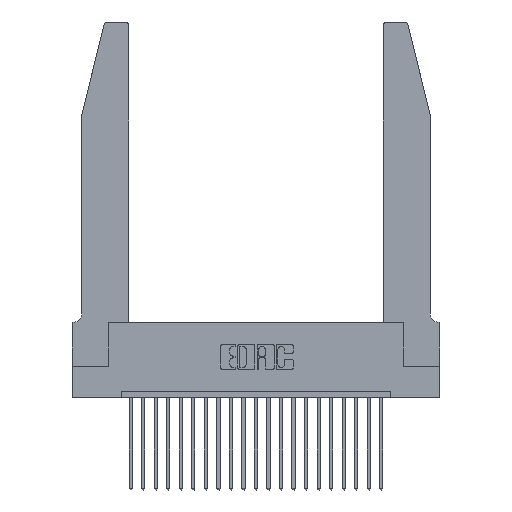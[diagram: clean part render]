
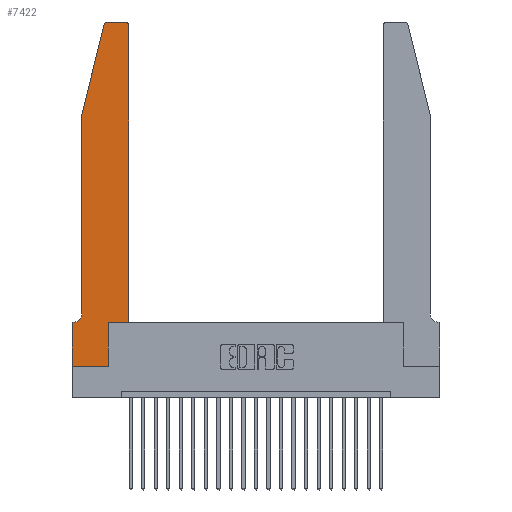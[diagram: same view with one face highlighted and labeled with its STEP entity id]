
A CAD part, top view. The second image highlights one B-rep face of the part: STEP entity #7422.
In plain terms, the highlighted planar face has unit normal (0, 0, 1).
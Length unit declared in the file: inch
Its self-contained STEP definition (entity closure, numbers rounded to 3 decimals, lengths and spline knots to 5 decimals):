
#168 = DIRECTION ( 'NONE',  ( 0., -1., 0. ) ) ;
#185 = VECTOR ( 'NONE', #168, 39.37008 ) ;
#1058 = CARTESIAN_POINT ( 'NONE',  ( 0., 0., 0.37 ) ) ;
#1091 = DIRECTION ( 'NONE',  ( 1., 0., 0. ) ) ;
#1201 = ORIENTED_EDGE ( 'NONE', *, *, #13110, .T. ) ;
#1692 = EDGE_CURVE ( 'NONE', #3059, #1806, #6596, .T. ) ;
#1806 = VERTEX_POINT ( 'NONE', #16091 ) ;
#1858 = CARTESIAN_POINT ( 'NONE',  ( 0.0055, 0.35, 0.37 ) ) ;
#1915 = VECTOR ( 'NONE', #3840, 39.37008 ) ;
#1952 = EDGE_LOOP ( 'NONE', ( #14640, #12118, #13056, #22120, #21061, #23394, #17642, #8916, #16453, #1201, #12430, #7201 ) ) ;
#1994 = AXIS2_PLACEMENT_3D ( 'NONE', #22771, #15600, #23003 ) ;
#2488 = EDGE_CURVE ( 'NONE', #17588, #18552, #19065, .T. ) ;
#2520 = AXIS2_PLACEMENT_3D ( 'NONE', #21531, #5009, #7047 ) ;
#3059 = VERTEX_POINT ( 'NONE', #19355 ) ;
#3170 = CIRCLE ( 'NONE', #3537, 0.03 ) ;
#3206 = VECTOR ( 'NONE', #23325, 39.37008 ) ;
#3537 = AXIS2_PLACEMENT_3D ( 'NONE', #4564, #6344, #1091 ) ;
#3687 = CARTESIAN_POINT ( 'NONE',  ( 0.2865, 0.35, 0.37 ) ) ;
#3840 = DIRECTION ( 'NONE',  ( -0.239, -0.971, 0. ) ) ;
#4564 = CARTESIAN_POINT ( 'NONE',  ( 0.284, 2.72, 0.37 ) ) ;
#4999 = LINE ( 'NONE', #12201, #185 ) ;
#5009 = DIRECTION ( 'NONE',  ( 0., 0., -1. ) ) ;
#5666 = DIRECTION ( 'NONE',  ( 1., 0., 0. ) ) ;
#5783 = PLANE ( 'NONE',  #11746 ) ;
#6344 = DIRECTION ( 'NONE',  ( 0., 0., 1. ) ) ;
#6596 = CIRCLE ( 'NONE', #1994, 0.03 ) ;
#6610 = VERTEX_POINT ( 'NONE', #14616 ) ;
#7047 = DIRECTION ( 'NONE',  ( -1., 0., 0. ) ) ;
#7201 = ORIENTED_EDGE ( 'NONE', *, *, #1692, .T. ) ;
#7284 = VERTEX_POINT ( 'NONE', #1858 ) ;
#7287 = CARTESIAN_POINT ( 'NONE',  ( 0.0755, 2., 0.37 ) ) ;
#7422 = ADVANCED_FACE ( 'NONE', ( #21648 ), #5783, .T. ) ;
#7629 = CARTESIAN_POINT ( 'NONE',  ( 0.2605, 2.75, 0.37 ) ) ;
#7743 = VECTOR ( 'NONE', #13198, 39.37008 ) ;
#8656 = LINE ( 'NONE', #7287, #1915 ) ;
#8835 = LINE ( 'NONE', #21524, #3206 ) ;
#8916 = ORIENTED_EDGE ( 'NONE', *, *, #15512, .T. ) ;
#9559 = CARTESIAN_POINT ( 'NONE',  ( 0., 0.35, 0.37 ) ) ;
#9866 = VECTOR ( 'NONE', #16115, 39.37008 ) ;
#10441 = CARTESIAN_POINT ( 'NONE',  ( 0.4505, 0.35, 0.37 ) ) ;
#10525 = EDGE_CURVE ( 'NONE', #16802, #6610, #4999, .T. ) ;
#11103 = EDGE_CURVE ( 'NONE', #19682, #16802, #8656, .T. ) ;
#11746 = AXIS2_PLACEMENT_3D ( 'NONE', #18501, #22245, #17152 ) ;
#12118 = ORIENTED_EDGE ( 'NONE', *, *, #17867, .T. ) ;
#12201 = CARTESIAN_POINT ( 'NONE',  ( 0.0755, 2., 0.37 ) ) ;
#12286 = CARTESIAN_POINT ( 'NONE',  ( 0.284, 2.75, 0.37 ) ) ;
#12384 = CARTESIAN_POINT ( 'NONE',  ( 0.0755, 0.35, 0.37 ) ) ;
#12430 = ORIENTED_EDGE ( 'NONE', *, *, #12512, .T. ) ;
#12512 = EDGE_CURVE ( 'NONE', #16644, #3059, #12854, .T. ) ;
#12854 = LINE ( 'NONE', #17814, #14546 ) ;
#12873 = CARTESIAN_POINT ( 'NONE',  ( 0.0755, 2., 0.37 ) ) ;
#12982 = CARTESIAN_POINT ( 'NONE',  ( 0.2865, 0., 0.37 ) ) ;
#13056 = ORIENTED_EDGE ( 'NONE', *, *, #11103, .T. ) ;
#13110 = EDGE_CURVE ( 'NONE', #13647, #16644, #8835, .T. ) ;
#13198 = DIRECTION ( 'NONE',  ( -1., 0., 0. ) ) ;
#13647 = VERTEX_POINT ( 'NONE', #14885 ) ;
#13722 = VECTOR ( 'NONE', #5666, 39.37008 ) ;
#13962 = LINE ( 'NONE', #7629, #7743 ) ;
#14505 = EDGE_CURVE ( 'NONE', #16985, #13647, #22277, .T. ) ;
#14546 = VECTOR ( 'NONE', #18055, 39.37008 ) ;
#14616 = CARTESIAN_POINT ( 'NONE',  ( 0.0755, 0.42, 0.37 ) ) ;
#14640 = ORIENTED_EDGE ( 'NONE', *, *, #16065, .T. ) ;
#14885 = CARTESIAN_POINT ( 'NONE',  ( 0.2865, 0.35, 0.37 ) ) ;
#15512 = EDGE_CURVE ( 'NONE', #18552, #16985, #23060, .T. ) ;
#15600 = DIRECTION ( 'NONE',  ( 0., 0., 1. ) ) ;
#15685 = DIRECTION ( 'NONE',  ( 0., -1., 0. ) ) ;
#16065 = EDGE_CURVE ( 'NONE', #1806, #20287, #13962, .T. ) ;
#16091 = CARTESIAN_POINT ( 'NONE',  ( 0.4205, 2.75, 0.37 ) ) ;
#16115 = DIRECTION ( 'NONE',  ( -1., 0., 0. ) ) ;
#16453 = ORIENTED_EDGE ( 'NONE', *, *, #14505, .T. ) ;
#16644 = VERTEX_POINT ( 'NONE', #10441 ) ;
#16802 = VERTEX_POINT ( 'NONE', #12873 ) ;
#16957 = VECTOR ( 'NONE', #19936, 39.37008 ) ;
#16985 = VERTEX_POINT ( 'NONE', #12982 ) ;
#17152 = DIRECTION ( 'NONE',  ( 1., 0., 0. ) ) ;
#17588 = VERTEX_POINT ( 'NONE', #9559 ) ;
#17642 = ORIENTED_EDGE ( 'NONE', *, *, #2488, .T. ) ;
#17814 = CARTESIAN_POINT ( 'NONE',  ( 0.4505, 0.35, 0.37 ) ) ;
#17833 = LINE ( 'NONE', #12384, #9866 ) ;
#17867 = EDGE_CURVE ( 'NONE', #20287, #19682, #3170, .T. ) ;
#18055 = DIRECTION ( 'NONE',  ( 0., 1., 0. ) ) ;
#18501 = CARTESIAN_POINT ( 'NONE',  ( 0., 0.35, 0.37 ) ) ;
#18552 = VERTEX_POINT ( 'NONE', #20846 ) ;
#18939 = EDGE_CURVE ( 'NONE', #6610, #7284, #21512, .T. ) ;
#19065 = LINE ( 'NONE', #1058, #22131 ) ;
#19355 = CARTESIAN_POINT ( 'NONE',  ( 0.4505, 2.72, 0.37 ) ) ;
#19682 = VERTEX_POINT ( 'NONE', #23054 ) ;
#19936 = DIRECTION ( 'NONE',  ( 0., 1., 0. ) ) ;
#20092 = EDGE_CURVE ( 'NONE', #7284, #17588, #17833, .T. ) ;
#20286 = CARTESIAN_POINT ( 'NONE',  ( 0., 0., 0.37 ) ) ;
#20287 = VERTEX_POINT ( 'NONE', #12286 ) ;
#20846 = CARTESIAN_POINT ( 'NONE',  ( 0., 0., 0.37 ) ) ;
#21061 = ORIENTED_EDGE ( 'NONE', *, *, #18939, .T. ) ;
#21512 = CIRCLE ( 'NONE', #2520, 0.07 ) ;
#21524 = CARTESIAN_POINT ( 'NONE',  ( 0.4505, 0.35, 0.37 ) ) ;
#21531 = CARTESIAN_POINT ( 'NONE',  ( 0.0055, 0.42, 0.37 ) ) ;
#21648 = FACE_OUTER_BOUND ( 'NONE', #1952, .T. ) ;
#22120 = ORIENTED_EDGE ( 'NONE', *, *, #10525, .T. ) ;
#22131 = VECTOR ( 'NONE', #15685, 39.37008 ) ;
#22245 = DIRECTION ( 'NONE',  ( 0., 0., 1. ) ) ;
#22277 = LINE ( 'NONE', #3687, #16957 ) ;
#22771 = CARTESIAN_POINT ( 'NONE',  ( 0.4205, 2.72, 0.37 ) ) ;
#23003 = DIRECTION ( 'NONE',  ( 1., 0., 0. ) ) ;
#23054 = CARTESIAN_POINT ( 'NONE',  ( 0.25487, 2.72718, 0.37 ) ) ;
#23060 = LINE ( 'NONE', #20286, #13722 ) ;
#23325 = DIRECTION ( 'NONE',  ( 1., 0., 0. ) ) ;
#23394 = ORIENTED_EDGE ( 'NONE', *, *, #20092, .T. ) ;
